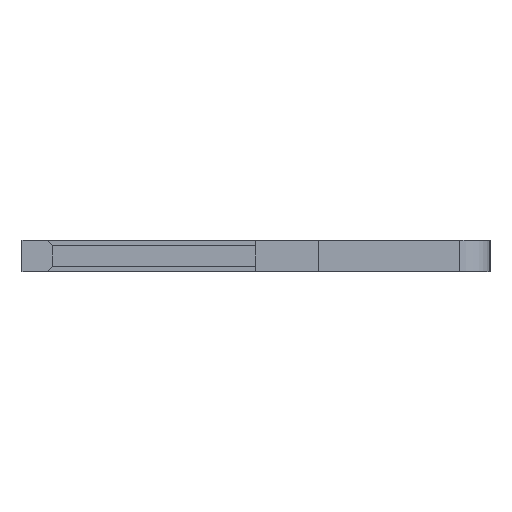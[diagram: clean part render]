
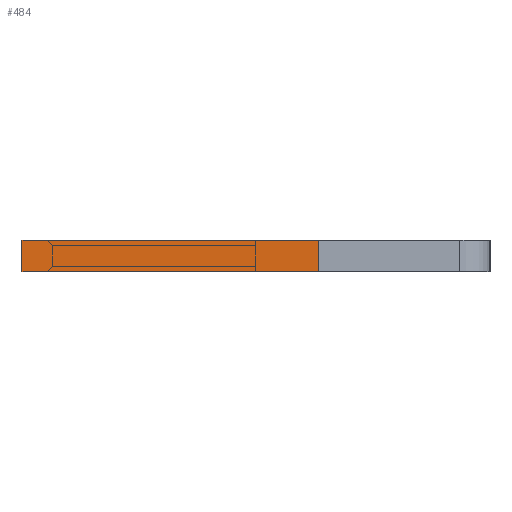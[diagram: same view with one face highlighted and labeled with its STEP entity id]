
A CAD part, left-side view. The second image highlights one B-rep face of the part: STEP entity #484.
In plain terms, the highlighted face is planar.
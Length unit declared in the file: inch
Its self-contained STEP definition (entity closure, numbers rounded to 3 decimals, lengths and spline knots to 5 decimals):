
#243 = VECTOR ( 'NONE', #2395, 39.37008 ) ;
#278 = AXIS2_PLACEMENT_3D ( 'NONE', #895, #3957, #1897 ) ;
#355 = CARTESIAN_POINT ( 'NONE',  ( -0.01, 0.15, -0.04 ) ) ;
#379 = LINE ( 'NONE', #3851, #3241 ) ;
#451 = DIRECTION ( 'NONE',  ( -1., 0., 0. ) ) ;
#484 = ADVANCED_FACE ( 'NONE', ( #1974 ), #1919, .F. ) ;
#492 = ORIENTED_EDGE ( 'NONE', *, *, #958, .T. ) ;
#742 = DIRECTION ( 'NONE',  ( 0., 1., 0. ) ) ;
#816 = ORIENTED_EDGE ( 'NONE', *, *, #2778, .F. ) ;
#832 = LINE ( 'NONE', #355, #243 ) ;
#895 = CARTESIAN_POINT ( 'NONE',  ( 0.01, 0.15, -0.04 ) ) ;
#958 = EDGE_CURVE ( 'NONE', #1396, #2149, #2617, .T. ) ;
#1339 = CARTESIAN_POINT ( 'NONE',  ( 0.01, -0.04, -0.04 ) ) ;
#1396 = VERTEX_POINT ( 'NONE', #1339 ) ;
#1729 = EDGE_CURVE ( 'NONE', #1396, #2139, #3126, .T. ) ;
#1897 = DIRECTION ( 'NONE',  ( 1., 0., 0. ) ) ;
#1919 = PLANE ( 'NONE',  #278 ) ;
#1974 = FACE_OUTER_BOUND ( 'NONE', #3353, .T. ) ;
#2026 = CARTESIAN_POINT ( 'NONE',  ( 0.01, 0.15, -0.04 ) ) ;
#2139 = VERTEX_POINT ( 'NONE', #4161 ) ;
#2143 = CARTESIAN_POINT ( 'NONE',  ( -0.01, -0.04, -0.04 ) ) ;
#2149 = VERTEX_POINT ( 'NONE', #2143 ) ;
#2395 = DIRECTION ( 'NONE',  ( 0., 1., 0. ) ) ;
#2571 = VECTOR ( 'NONE', #3673, 39.37008 ) ;
#2617 = LINE ( 'NONE', #3346, #2571 ) ;
#2723 = ORIENTED_EDGE ( 'NONE', *, *, #2849, .T. ) ;
#2778 = EDGE_CURVE ( 'NONE', #2139, #3311, #379, .T. ) ;
#2849 = EDGE_CURVE ( 'NONE', #2149, #3311, #832, .T. ) ;
#2876 = VECTOR ( 'NONE', #742, 39.37008 ) ;
#3126 = LINE ( 'NONE', #2026, #2876 ) ;
#3241 = VECTOR ( 'NONE', #451, 39.37008 ) ;
#3311 = VERTEX_POINT ( 'NONE', #3669 ) ;
#3346 = CARTESIAN_POINT ( 'NONE',  ( 0.01, -0.04, -0.04 ) ) ;
#3353 = EDGE_LOOP ( 'NONE', ( #2723, #816, #4070, #492 ) ) ;
#3669 = CARTESIAN_POINT ( 'NONE',  ( -0.01, 0.15, -0.04 ) ) ;
#3673 = DIRECTION ( 'NONE',  ( -1., 0., 0. ) ) ;
#3851 = CARTESIAN_POINT ( 'NONE',  ( 0.01, 0.15, -0.04 ) ) ;
#3957 = DIRECTION ( 'NONE',  ( 0., 0., 1. ) ) ;
#4070 = ORIENTED_EDGE ( 'NONE', *, *, #1729, .F. ) ;
#4161 = CARTESIAN_POINT ( 'NONE',  ( 0.01, 0.15, -0.04 ) ) ;
